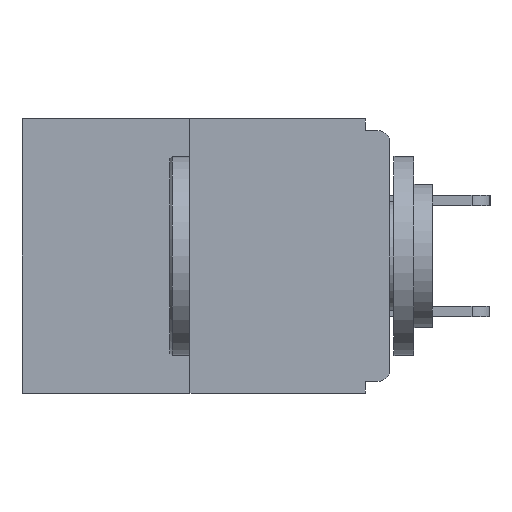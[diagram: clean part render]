
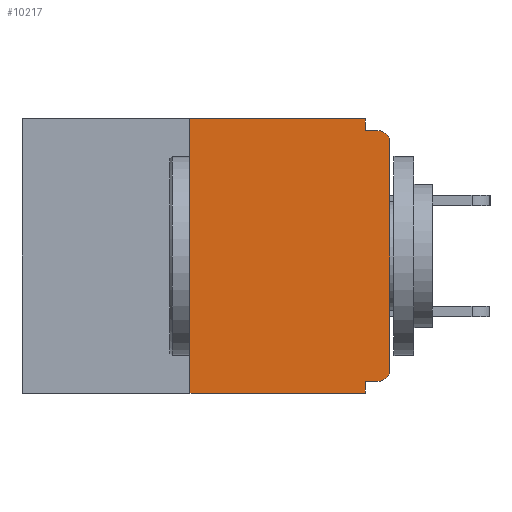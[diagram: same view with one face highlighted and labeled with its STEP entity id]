
A CAD part, left-side view. The second image highlights one B-rep face of the part: STEP entity #10217.
In plain terms, the highlighted planar face has unit normal (-1, 0, 0).
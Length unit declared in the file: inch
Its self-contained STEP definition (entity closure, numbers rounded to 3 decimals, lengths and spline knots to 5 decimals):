
#46 = DIRECTION ( 'NONE',  ( 0., 0., 1. ) ) ;
#180 = DIRECTION ( 'NONE',  ( 0., 0., -1. ) ) ;
#182 = ORIENTED_EDGE ( 'NONE', *, *, #3210, .F. ) ;
#549 = VECTOR ( 'NONE', #46, 39.37008 ) ;
#573 = AXIS2_PLACEMENT_3D ( 'NONE', #11699, #1230, #6134 ) ;
#602 = VECTOR ( 'NONE', #180, 39.37008 ) ;
#687 = VECTOR ( 'NONE', #8758, 39.37008 ) ;
#1135 = EDGE_CURVE ( 'NONE', #4542, #2875, #3520, .T. ) ;
#1164 = EDGE_CURVE ( 'NONE', #12371, #4987, #7207, .T. ) ;
#1182 = ORIENTED_EDGE ( 'NONE', *, *, #9632, .F. ) ;
#1230 = DIRECTION ( 'NONE',  ( 1., 0., 0. ) ) ;
#2059 = LINE ( 'NONE', #4667, #12195 ) ;
#2064 = CARTESIAN_POINT ( 'NONE',  ( 0., 0.25, 0. ) ) ;
#2131 = CARTESIAN_POINT ( 'NONE',  ( 0., 0., -0.03 ) ) ;
#2362 = CARTESIAN_POINT ( 'NONE',  ( 0., 0.015, -0.015 ) ) ;
#2450 = VECTOR ( 'NONE', #12018, 39.37008 ) ;
#2489 = AXIS2_PLACEMENT_3D ( 'NONE', #8867, #9990, #12021 ) ;
#2609 = CARTESIAN_POINT ( 'NONE',  ( 0., 0.25, -0.343 ) ) ;
#2754 = EDGE_CURVE ( 'NONE', #5319, #12371, #10226, .T. ) ;
#2875 = VERTEX_POINT ( 'NONE', #11014 ) ;
#3005 = CARTESIAN_POINT ( 'NONE',  ( 0., 0.015, -0.313 ) ) ;
#3109 = VECTOR ( 'NONE', #7378, 39.37008 ) ;
#3210 = EDGE_CURVE ( 'NONE', #11371, #5528, #9278, .T. ) ;
#3212 = DIRECTION ( 'NONE',  ( 0., 0., -1. ) ) ;
#3413 = VECTOR ( 'NONE', #8900, 39.37008 ) ;
#3520 = LINE ( 'NONE', #11931, #602 ) ;
#4000 = CARTESIAN_POINT ( 'NONE',  ( 0., 0., 0. ) ) ;
#4027 = LINE ( 'NONE', #2064, #3413 ) ;
#4437 = CARTESIAN_POINT ( 'NONE',  ( 0., 0.25, 0. ) ) ;
#4449 = CARTESIAN_POINT ( 'NONE',  ( 0., 0.031, -0.343 ) ) ;
#4542 = VERTEX_POINT ( 'NONE', #8331 ) ;
#4667 = CARTESIAN_POINT ( 'NONE',  ( 0., 0., -0.015 ) ) ;
#4852 = CARTESIAN_POINT ( 'NONE',  ( 0., 0.46, 0. ) ) ;
#4987 = VERTEX_POINT ( 'NONE', #2362 ) ;
#5058 = LINE ( 'NONE', #10031, #2450 ) ;
#5151 = ORIENTED_EDGE ( 'NONE', *, *, #6852, .F. ) ;
#5211 = EDGE_CURVE ( 'NONE', #2875, #4987, #2059, .T. ) ;
#5319 = VERTEX_POINT ( 'NONE', #9094 ) ;
#5528 = VERTEX_POINT ( 'NONE', #11933 ) ;
#5588 = CARTESIAN_POINT ( 'NONE',  ( 0., 0.031, -0.343 ) ) ;
#5734 = ORIENTED_EDGE ( 'NONE', *, *, #5211, .F. ) ;
#5871 = DIRECTION ( 'NONE',  ( 0., -1., 0. ) ) ;
#5953 = ORIENTED_EDGE ( 'NONE', *, *, #2754, .T. ) ;
#6049 = LINE ( 'NONE', #4449, #3109 ) ;
#6134 = DIRECTION ( 'NONE',  ( 0., 0., -1. ) ) ;
#6320 = AXIS2_PLACEMENT_3D ( 'NONE', #3005, #10114, #3212 ) ;
#6562 = CARTESIAN_POINT ( 'NONE',  ( 0., 0., -0.328 ) ) ;
#6852 = EDGE_CURVE ( 'NONE', #10105, #4542, #10884, .T. ) ;
#7207 = CIRCLE ( 'NONE', #2489, 0.015 ) ;
#7312 = CIRCLE ( 'NONE', #6320, 0.015 ) ;
#7378 = DIRECTION ( 'NONE',  ( 0., 0., -1. ) ) ;
#7432 = EDGE_CURVE ( 'NONE', #11371, #5319, #7312, .T. ) ;
#7649 = DIRECTION ( 'NONE',  ( 0., -1., 0. ) ) ;
#7769 = CARTESIAN_POINT ( 'NONE',  ( 0., 0.015, -0.328 ) ) ;
#8121 = VERTEX_POINT ( 'NONE', #5588 ) ;
#8277 = ORIENTED_EDGE ( 'NONE', *, *, #7432, .T. ) ;
#8331 = CARTESIAN_POINT ( 'NONE',  ( 0., 0.031, 0. ) ) ;
#8465 = FACE_OUTER_BOUND ( 'NONE', #12611, .T. ) ;
#8633 = PLANE ( 'NONE',  #573 ) ;
#8695 = ORIENTED_EDGE ( 'NONE', *, *, #9859, .F. ) ;
#8758 = DIRECTION ( 'NONE',  ( 0., 1., 0. ) ) ;
#8867 = CARTESIAN_POINT ( 'NONE',  ( 0., 0.015, -0.03 ) ) ;
#8900 = DIRECTION ( 'NONE',  ( 0., 0., 1. ) ) ;
#9094 = CARTESIAN_POINT ( 'NONE',  ( 0., 0., -0.313 ) ) ;
#9174 = ORIENTED_EDGE ( 'NONE', *, *, #1135, .F. ) ;
#9278 = LINE ( 'NONE', #6562, #687 ) ;
#9557 = ORIENTED_EDGE ( 'NONE', *, *, #1164, .T. ) ;
#9632 = EDGE_CURVE ( 'NONE', #5528, #8121, #6049, .T. ) ;
#9859 = EDGE_CURVE ( 'NONE', #11126, #10105, #4027, .T. ) ;
#9990 = DIRECTION ( 'NONE',  ( -1., 0., 0. ) ) ;
#10031 = CARTESIAN_POINT ( 'NONE',  ( 0., 0.46, -0.343 ) ) ;
#10105 = VERTEX_POINT ( 'NONE', #4437 ) ;
#10114 = DIRECTION ( 'NONE',  ( -1., 0., 0. ) ) ;
#10217 = ADVANCED_FACE ( 'NONE', ( #8465 ), #8633, .F. ) ;
#10226 = LINE ( 'NONE', #4000, #549 ) ;
#10491 = ORIENTED_EDGE ( 'NONE', *, *, #12700, .T. ) ;
#10884 = LINE ( 'NONE', #4852, #12460 ) ;
#11014 = CARTESIAN_POINT ( 'NONE',  ( 0., 0.031, -0.015 ) ) ;
#11126 = VERTEX_POINT ( 'NONE', #2609 ) ;
#11371 = VERTEX_POINT ( 'NONE', #7769 ) ;
#11699 = CARTESIAN_POINT ( 'NONE',  ( 0., 0.46, 0. ) ) ;
#11931 = CARTESIAN_POINT ( 'NONE',  ( 0., 0.031, 0. ) ) ;
#11933 = CARTESIAN_POINT ( 'NONE',  ( 0., 0.031, -0.328 ) ) ;
#12018 = DIRECTION ( 'NONE',  ( 0., -1., 0. ) ) ;
#12021 = DIRECTION ( 'NONE',  ( 0., 0., -1. ) ) ;
#12195 = VECTOR ( 'NONE', #7649, 39.37008 ) ;
#12371 = VERTEX_POINT ( 'NONE', #2131 ) ;
#12460 = VECTOR ( 'NONE', #5871, 39.37008 ) ;
#12611 = EDGE_LOOP ( 'NONE', ( #5151, #8695, #10491, #1182, #182, #8277, #5953, #9557, #5734, #9174 ) ) ;
#12700 = EDGE_CURVE ( 'NONE', #11126, #8121, #5058, .T. ) ;
